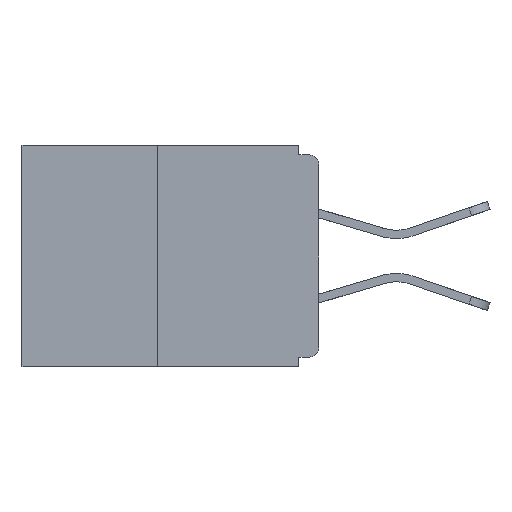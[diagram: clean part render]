
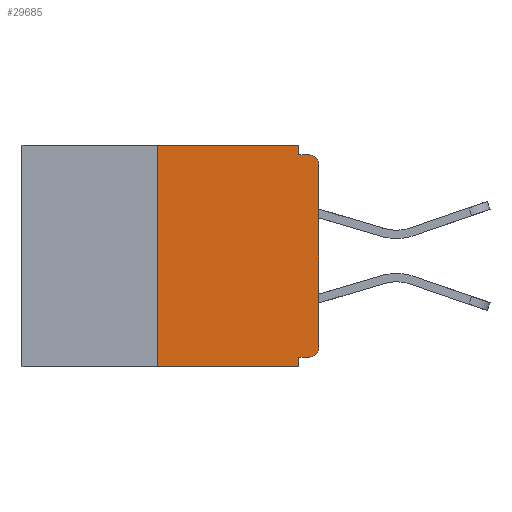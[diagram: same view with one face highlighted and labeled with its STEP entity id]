
A CAD part, left-side view. The second image highlights one B-rep face of the part: STEP entity #29685.
In plain terms, the highlighted planar face has unit normal (-1, 0, 0).
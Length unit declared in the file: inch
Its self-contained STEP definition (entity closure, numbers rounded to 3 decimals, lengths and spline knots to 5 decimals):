
#159 = ORIENTED_EDGE ( 'NONE', *, *, #20563, .F. ) ;
#432 = CARTESIAN_POINT ( 'NONE',  ( 0., 0., 0. ) ) ;
#1899 = CIRCLE ( 'NONE', #10801, 0.015 ) ;
#2004 = CARTESIAN_POINT ( 'NONE',  ( 0., 0.46, 0. ) ) ;
#2200 = CARTESIAN_POINT ( 'NONE',  ( 0., 0.031, -0.015 ) ) ;
#2341 = VERTEX_POINT ( 'NONE', #26035 ) ;
#2949 = ORIENTED_EDGE ( 'NONE', *, *, #9367, .T. ) ;
#3300 = EDGE_CURVE ( 'NONE', #23761, #27076, #12655, .T. ) ;
#3762 = CARTESIAN_POINT ( 'NONE',  ( 0., 0.031, -0.328 ) ) ;
#3861 = CIRCLE ( 'NONE', #29043, 0.015 ) ;
#4042 = PLANE ( 'NONE',  #19796 ) ;
#4191 = LINE ( 'NONE', #7169, #10412 ) ;
#4447 = CARTESIAN_POINT ( 'NONE',  ( 0., 0.031, -0.343 ) ) ;
#4479 = CARTESIAN_POINT ( 'NONE',  ( 0., 0., -0.03 ) ) ;
#4811 = LINE ( 'NONE', #28609, #13941 ) ;
#5143 = ORIENTED_EDGE ( 'NONE', *, *, #5729, .T. ) ;
#5207 = CARTESIAN_POINT ( 'NONE',  ( 0., 0.015, -0.03 ) ) ;
#5225 = LINE ( 'NONE', #27201, #15782 ) ;
#5319 = ORIENTED_EDGE ( 'NONE', *, *, #12255, .T. ) ;
#5562 = VERTEX_POINT ( 'NONE', #4479 ) ;
#5729 = EDGE_CURVE ( 'NONE', #13981, #28245, #1899, .T. ) ;
#6449 = CARTESIAN_POINT ( 'NONE',  ( 0., 0.031, 0. ) ) ;
#6740 = VECTOR ( 'NONE', #18794, 39.37008 ) ;
#7169 = CARTESIAN_POINT ( 'NONE',  ( 0., 0.46, 0. ) ) ;
#9279 = EDGE_CURVE ( 'NONE', #2341, #11108, #4191, .T. ) ;
#9367 = EDGE_CURVE ( 'NONE', #28834, #28822, #17702, .T. ) ;
#10296 = CARTESIAN_POINT ( 'NONE',  ( 0., 0.031, -0.343 ) ) ;
#10412 = VECTOR ( 'NONE', #26015, 39.37008 ) ;
#10769 = LINE ( 'NONE', #10296, #28270 ) ;
#10801 = AXIS2_PLACEMENT_3D ( 'NONE', #13429, #29444, #29539 ) ;
#11108 = VERTEX_POINT ( 'NONE', #6449 ) ;
#11688 = CARTESIAN_POINT ( 'NONE',  ( 0., 0.25, -0.343 ) ) ;
#11825 = DIRECTION ( 'NONE',  ( 0., 0., 1. ) ) ;
#12143 = ORIENTED_EDGE ( 'NONE', *, *, #12878, .F. ) ;
#12255 = EDGE_CURVE ( 'NONE', #5562, #27076, #3861, .T. ) ;
#12514 = ORIENTED_EDGE ( 'NONE', *, *, #3300, .F. ) ;
#12655 = LINE ( 'NONE', #13940, #22518 ) ;
#12719 = DIRECTION ( 'NONE',  ( 0., 0., -1. ) ) ;
#12835 = EDGE_CURVE ( 'NONE', #28245, #5562, #14774, .T. ) ;
#12878 = EDGE_CURVE ( 'NONE', #27807, #28822, #10769, .T. ) ;
#13029 = FACE_OUTER_BOUND ( 'NONE', #23884, .T. ) ;
#13429 = CARTESIAN_POINT ( 'NONE',  ( 0., 0.015, -0.313 ) ) ;
#13940 = CARTESIAN_POINT ( 'NONE',  ( 0., 0., -0.015 ) ) ;
#13941 = VECTOR ( 'NONE', #12719, 39.37008 ) ;
#13981 = VERTEX_POINT ( 'NONE', #18788 ) ;
#14774 = LINE ( 'NONE', #432, #27919 ) ;
#15782 = VECTOR ( 'NONE', #26551, 39.37008 ) ;
#16604 = DIRECTION ( 'NONE',  ( 0., -1., 0. ) ) ;
#16776 = DIRECTION ( 'NONE',  ( 0., 0., 1. ) ) ;
#17092 = ORIENTED_EDGE ( 'NONE', *, *, #9279, .F. ) ;
#17702 = LINE ( 'NONE', #21435, #6740 ) ;
#18788 = CARTESIAN_POINT ( 'NONE',  ( 0., 0.015, -0.328 ) ) ;
#18794 = DIRECTION ( 'NONE',  ( 0., -1., 0. ) ) ;
#18984 = DIRECTION ( 'NONE',  ( 0., 0., -1. ) ) ;
#19559 = LINE ( 'NONE', #21175, #25359 ) ;
#19796 = AXIS2_PLACEMENT_3D ( 'NONE', #2004, #25275, #25163 ) ;
#19968 = ORIENTED_EDGE ( 'NONE', *, *, #12835, .T. ) ;
#20563 = EDGE_CURVE ( 'NONE', #28834, #2341, #19559, .T. ) ;
#20602 = CARTESIAN_POINT ( 'NONE',  ( 0., 0.015, -0.015 ) ) ;
#21175 = CARTESIAN_POINT ( 'NONE',  ( 0., 0.25, 0. ) ) ;
#21435 = CARTESIAN_POINT ( 'NONE',  ( 0., 0.46, -0.343 ) ) ;
#21606 = ORIENTED_EDGE ( 'NONE', *, *, #25911, .F. ) ;
#21634 = ORIENTED_EDGE ( 'NONE', *, *, #22287, .F. ) ;
#21851 = DIRECTION ( 'NONE',  ( 0., 0., -1. ) ) ;
#22287 = EDGE_CURVE ( 'NONE', #13981, #27807, #5225, .T. ) ;
#22518 = VECTOR ( 'NONE', #16604, 39.37008 ) ;
#23571 = CARTESIAN_POINT ( 'NONE',  ( 0., 0., -0.313 ) ) ;
#23761 = VERTEX_POINT ( 'NONE', #2200 ) ;
#23884 = EDGE_LOOP ( 'NONE', ( #17092, #159, #2949, #12143, #21634, #5143, #19968, #5319, #12514, #21606 ) ) ;
#25163 = DIRECTION ( 'NONE',  ( 0., 0., -1. ) ) ;
#25275 = DIRECTION ( 'NONE',  ( 1., 0., 0. ) ) ;
#25359 = VECTOR ( 'NONE', #16776, 39.37008 ) ;
#25911 = EDGE_CURVE ( 'NONE', #11108, #23761, #4811, .T. ) ;
#26015 = DIRECTION ( 'NONE',  ( 0., -1., 0. ) ) ;
#26035 = CARTESIAN_POINT ( 'NONE',  ( 0., 0.25, 0. ) ) ;
#26104 = DIRECTION ( 'NONE',  ( -1., 0., 0. ) ) ;
#26551 = DIRECTION ( 'NONE',  ( 0., 1., 0. ) ) ;
#27076 = VERTEX_POINT ( 'NONE', #20602 ) ;
#27201 = CARTESIAN_POINT ( 'NONE',  ( 0., 0., -0.328 ) ) ;
#27807 = VERTEX_POINT ( 'NONE', #3762 ) ;
#27919 = VECTOR ( 'NONE', #11825, 39.37008 ) ;
#28245 = VERTEX_POINT ( 'NONE', #23571 ) ;
#28270 = VECTOR ( 'NONE', #21851, 39.37008 ) ;
#28609 = CARTESIAN_POINT ( 'NONE',  ( 0., 0.031, 0. ) ) ;
#28822 = VERTEX_POINT ( 'NONE', #4447 ) ;
#28834 = VERTEX_POINT ( 'NONE', #11688 ) ;
#29043 = AXIS2_PLACEMENT_3D ( 'NONE', #5207, #26104, #18984 ) ;
#29444 = DIRECTION ( 'NONE',  ( -1., 0., 0. ) ) ;
#29539 = DIRECTION ( 'NONE',  ( 0., 0., -1. ) ) ;
#29685 = ADVANCED_FACE ( 'NONE', ( #13029 ), #4042, .F. ) ;
